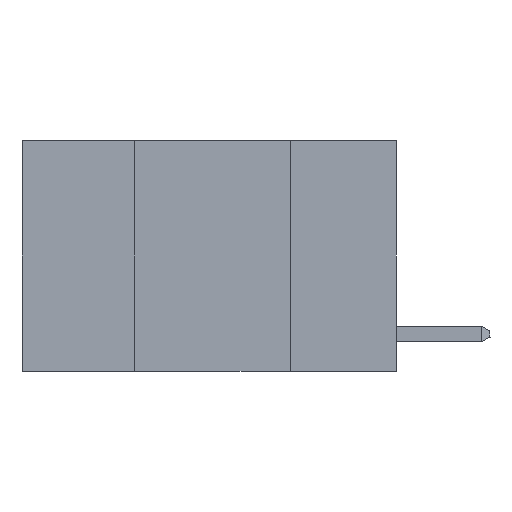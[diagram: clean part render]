
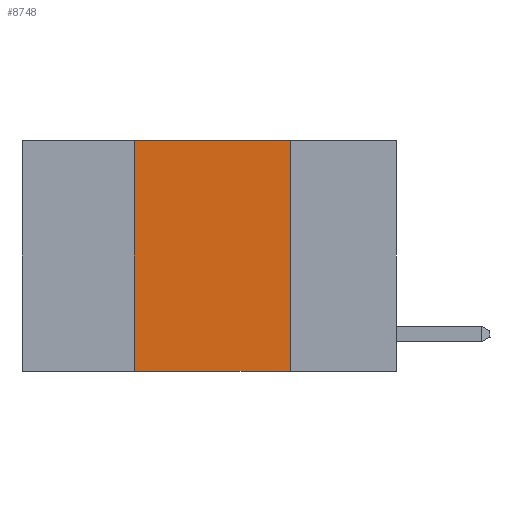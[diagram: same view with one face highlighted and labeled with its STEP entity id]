
A CAD part, left-side view. The second image highlights one B-rep face of the part: STEP entity #8748.
In plain terms, the highlighted planar face has unit normal (-1, 0, 0).
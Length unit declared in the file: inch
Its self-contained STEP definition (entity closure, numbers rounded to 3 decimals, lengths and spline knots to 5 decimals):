
#378 = ORIENTED_EDGE ( 'NONE', *, *, #24078, .F. ) ;
#1246 = EDGE_CURVE ( 'NONE', #12153, #13474, #29262, .T. ) ;
#2132 = ORIENTED_EDGE ( 'NONE', *, *, #21755, .F. ) ;
#3039 = FACE_OUTER_BOUND ( 'NONE', #29940, .T. ) ;
#3939 = CARTESIAN_POINT ( 'NONE',  ( 0., 0.17, 0. ) ) ;
#4248 = DIRECTION ( 'NONE',  ( 0., 0., -1. ) ) ;
#5428 = ORIENTED_EDGE ( 'NONE', *, *, #17746, .T. ) ;
#5429 = VECTOR ( 'NONE', #14871, 39.37008 ) ;
#6831 = CARTESIAN_POINT ( 'NONE',  ( 0., 0.42, 0. ) ) ;
#7240 = LINE ( 'NONE', #8065, #5429 ) ;
#8065 = CARTESIAN_POINT ( 'NONE',  ( 0., 0.6, -0.37 ) ) ;
#8597 = AXIS2_PLACEMENT_3D ( 'NONE', #27098, #12517, #24650 ) ;
#8748 = ADVANCED_FACE ( 'NONE', ( #3039 ), #22414, .F. ) ;
#9784 = CARTESIAN_POINT ( 'NONE',  ( 0., 0.6, 0. ) ) ;
#12153 = VERTEX_POINT ( 'NONE', #20373 ) ;
#12420 = VECTOR ( 'NONE', #14758, 39.37008 ) ;
#12517 = DIRECTION ( 'NONE',  ( 1., 0., 0. ) ) ;
#12875 = VECTOR ( 'NONE', #23278, 39.37008 ) ;
#13474 = VERTEX_POINT ( 'NONE', #16306 ) ;
#14758 = DIRECTION ( 'NONE',  ( 0., -1., 0. ) ) ;
#14871 = DIRECTION ( 'NONE',  ( 0., -1., 0. ) ) ;
#15404 = ORIENTED_EDGE ( 'NONE', *, *, #1246, .F. ) ;
#16306 = CARTESIAN_POINT ( 'NONE',  ( 0., 0.42, 0. ) ) ;
#17562 = VERTEX_POINT ( 'NONE', #20723 ) ;
#17746 = EDGE_CURVE ( 'NONE', #12153, #21664, #7240, .T. ) ;
#20373 = CARTESIAN_POINT ( 'NONE',  ( 0., 0.42, -0.37 ) ) ;
#20723 = CARTESIAN_POINT ( 'NONE',  ( 0., 0.17, 0. ) ) ;
#21664 = VERTEX_POINT ( 'NONE', #27234 ) ;
#21755 = EDGE_CURVE ( 'NONE', #17562, #21664, #24949, .T. ) ;
#22414 = PLANE ( 'NONE',  #8597 ) ;
#23278 = DIRECTION ( 'NONE',  ( 0., 0., 1. ) ) ;
#24078 = EDGE_CURVE ( 'NONE', #13474, #17562, #28802, .T. ) ;
#24650 = DIRECTION ( 'NONE',  ( 0., 0., -1. ) ) ;
#24949 = LINE ( 'NONE', #3939, #29311 ) ;
#27098 = CARTESIAN_POINT ( 'NONE',  ( 0., 0.6, 0. ) ) ;
#27234 = CARTESIAN_POINT ( 'NONE',  ( 0., 0.17, -0.37 ) ) ;
#28802 = LINE ( 'NONE', #9784, #12420 ) ;
#29262 = LINE ( 'NONE', #6831, #12875 ) ;
#29311 = VECTOR ( 'NONE', #4248, 39.37008 ) ;
#29940 = EDGE_LOOP ( 'NONE', ( #2132, #378, #15404, #5428 ) ) ;
